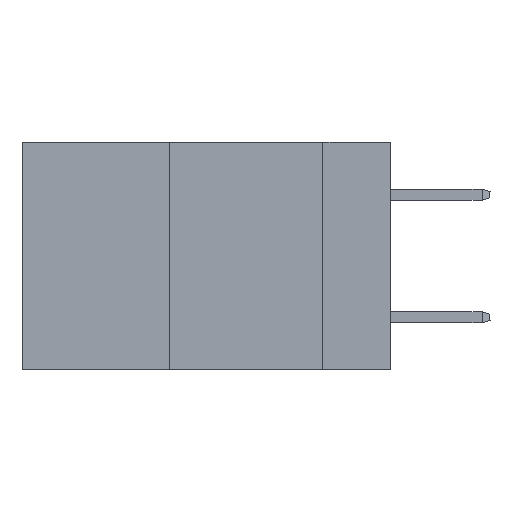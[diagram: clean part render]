
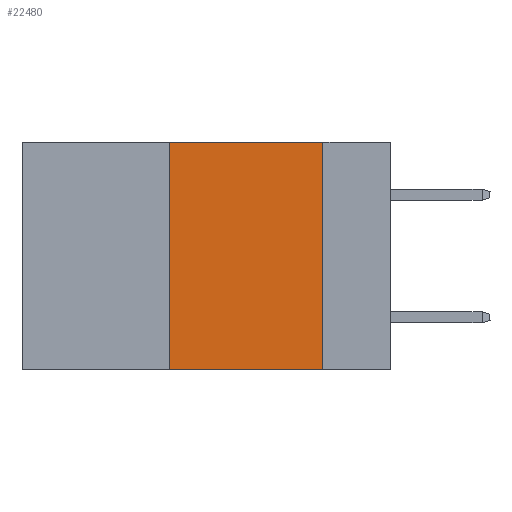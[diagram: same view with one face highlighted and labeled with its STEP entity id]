
A CAD part, left-side view. The second image highlights one B-rep face of the part: STEP entity #22480.
In plain terms, the highlighted planar face has unit normal (-1, 0, 0).
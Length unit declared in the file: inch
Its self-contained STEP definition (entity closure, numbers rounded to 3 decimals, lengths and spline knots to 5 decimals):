
#289 = ORIENTED_EDGE ( 'NONE', *, *, #38343, .F. ) ;
#1420 = LINE ( 'NONE', #20073, #20478 ) ;
#2930 = CARTESIAN_POINT ( 'NONE',  ( 0., 0.36, -0.37 ) ) ;
#3048 = LINE ( 'NONE', #35748, #33656 ) ;
#4725 = AXIS2_PLACEMENT_3D ( 'NONE', #12000, #23655, #32364 ) ;
#4754 = LINE ( 'NONE', #5751, #34429 ) ;
#5751 = CARTESIAN_POINT ( 'NONE',  ( 0., 0.11, 0. ) ) ;
#6547 = DIRECTION ( 'NONE',  ( 0., 0., 1. ) ) ;
#7294 = EDGE_CURVE ( 'NONE', #16571, #24002, #1420, .T. ) ;
#7351 = VERTEX_POINT ( 'NONE', #2930 ) ;
#8965 = VECTOR ( 'NONE', #6547, 39.37008 ) ;
#9033 = ORIENTED_EDGE ( 'NONE', *, *, #13817, .F. ) ;
#9448 = LINE ( 'NONE', #15415, #8965 ) ;
#12000 = CARTESIAN_POINT ( 'NONE',  ( 0., 0.6, 0. ) ) ;
#13817 = EDGE_CURVE ( 'NONE', #24002, #28092, #4754, .T. ) ;
#15415 = CARTESIAN_POINT ( 'NONE',  ( 0., 0.36, 0. ) ) ;
#16571 = VERTEX_POINT ( 'NONE', #34527 ) ;
#17431 = EDGE_CURVE ( 'NONE', #7351, #28092, #3048, .T. ) ;
#18159 = DIRECTION ( 'NONE',  ( 0., -1., 0. ) ) ;
#20073 = CARTESIAN_POINT ( 'NONE',  ( 0., 0.6, 0. ) ) ;
#20478 = VECTOR ( 'NONE', #31969, 39.37008 ) ;
#22480 = ADVANCED_FACE ( 'NONE', ( #25630 ), #38292, .F. ) ;
#23655 = DIRECTION ( 'NONE',  ( 1., 0., 0. ) ) ;
#23782 = DIRECTION ( 'NONE',  ( 0., 0., -1. ) ) ;
#24002 = VERTEX_POINT ( 'NONE', #35276 ) ;
#24276 = CARTESIAN_POINT ( 'NONE',  ( 0., 0.11, -0.37 ) ) ;
#25630 = FACE_OUTER_BOUND ( 'NONE', #27345, .T. ) ;
#27345 = EDGE_LOOP ( 'NONE', ( #9033, #33977, #289, #34587 ) ) ;
#28092 = VERTEX_POINT ( 'NONE', #24276 ) ;
#31969 = DIRECTION ( 'NONE',  ( 0., -1., 0. ) ) ;
#32364 = DIRECTION ( 'NONE',  ( 0., 0., -1. ) ) ;
#33656 = VECTOR ( 'NONE', #18159, 39.37008 ) ;
#33977 = ORIENTED_EDGE ( 'NONE', *, *, #7294, .F. ) ;
#34429 = VECTOR ( 'NONE', #23782, 39.37008 ) ;
#34527 = CARTESIAN_POINT ( 'NONE',  ( 0., 0.36, 0. ) ) ;
#34587 = ORIENTED_EDGE ( 'NONE', *, *, #17431, .T. ) ;
#35276 = CARTESIAN_POINT ( 'NONE',  ( 0., 0.11, 0. ) ) ;
#35748 = CARTESIAN_POINT ( 'NONE',  ( 0., 0.6, -0.37 ) ) ;
#38292 = PLANE ( 'NONE',  #4725 ) ;
#38343 = EDGE_CURVE ( 'NONE', #7351, #16571, #9448, .T. ) ;
